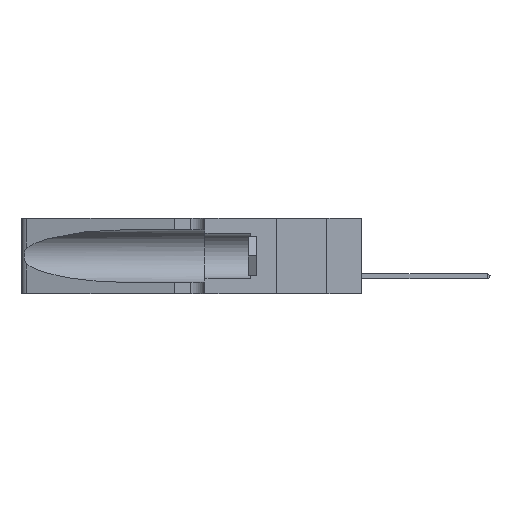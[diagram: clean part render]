
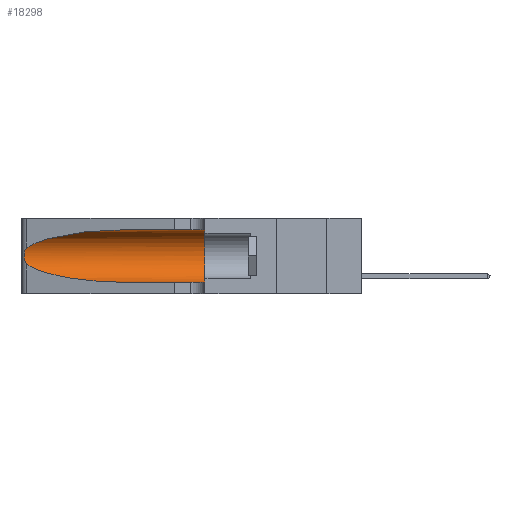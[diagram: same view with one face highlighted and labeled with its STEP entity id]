
A CAD part, left-side view. The second image highlights one B-rep face of the part: STEP entity #18298.
In plain terms, the highlighted cylindrical face has radius 3.308 mm (diameter 6.617 mm), a partial arc.
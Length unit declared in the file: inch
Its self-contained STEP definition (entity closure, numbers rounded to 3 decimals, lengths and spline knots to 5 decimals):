
#325 = DIRECTION ( 'NONE',  ( 0., -1., 0. ) ) ;
#591 = DIRECTION ( 'NONE',  ( 0., 1., 0. ) ) ;
#766 = ORIENTED_EDGE ( 'NONE', *, *, #35172, .T. ) ;
#852 = CARTESIAN_POINT ( 'NONE',  ( 0.25787, 1.23484, 0.2124 ) ) ;
#1067 = CARTESIAN_POINT ( 'NONE',  ( 0.1305, 1.61858, 0.05475 ) ) ;
#1559 = DIRECTION ( 'NONE',  ( 0., -1., 0. ) ) ;
#2289 = VERTEX_POINT ( 'NONE', #9120 ) ;
#2767 = CARTESIAN_POINT ( 'NONE',  ( 0.1305, 1.61858, 0.185 ) ) ;
#3626 = CARTESIAN_POINT ( 'NONE',  ( 0.25856, 1.23593, 0.16098 ) ) ;
#3762 = CARTESIAN_POINT ( 'NONE',  ( 0.25555, 1.22993, 0.14849 ) ) ;
#3997 = CARTESIAN_POINT ( 'NONE',  ( 0.25487, 1.22718, 0.14631 ) ) ;
#4197 = CARTESIAN_POINT ( 'NONE',  ( 0.25487, 1.22718, 0.22369 ) ) ;
#5621 = B_SPLINE_CURVE_WITH_KNOTS ( 'NONE', 3,
 ( #35063, #23959, #24080, #852, #24212, #26990, #6824, #27115, #29912, #3626, #15355, #6574, #3762, #3997 ),
 .UNSPECIFIED., .F., .F.,
 ( 4, 2, 2, 2, 2, 2, 4 ),
 ( 0., 0.00027, 0.00053, 0.00107, 0.0016, 0.00187, 0.00214 ),
 .UNSPECIFIED. ) ;
#6574 = CARTESIAN_POINT ( 'NONE',  ( 0.25639, 1.23186, 0.15144 ) ) ;
#6824 = CARTESIAN_POINT ( 'NONE',  ( 0.26075, 1.23896, 0.19203 ) ) ;
#7132 = CARTESIAN_POINT ( 'NONE',  ( 0.18966, 0.96281, 0.31525 ) ) ;
#7802 = ORIENTED_EDGE ( 'NONE', *, *, #27422, .F. ) ;
#8038 = CARTESIAN_POINT ( 'NONE',  ( 0.25487, 1.22718, 0.14631 ) ) ;
#8056 = LINE ( 'NONE', #1067, #30304 ) ;
#8158 = CARTESIAN_POINT ( 'NONE',  ( 0.1305, 0.72297, 0.05475 ) ) ;
#9120 = CARTESIAN_POINT ( 'NONE',  ( 0.1305, 0.72297, 0.05475 ) ) ;
#9625 = AXIS2_PLACEMENT_3D ( 'NONE', #2767, #325, #32314 ) ;
#10838 = CARTESIAN_POINT ( 'NONE',  ( 0.18966, 0.96281, 0.05475 ) ) ;
#10962 = CARTESIAN_POINT ( 'NONE',  ( 0.2373, 1.15595, 0.08982 ) ) ;
#11157 = EDGE_CURVE ( 'NONE', #15768, #31867, #32030, .T. ) ;
#11395 = VERTEX_POINT ( 'NONE', #28907 ) ;
#12294 = DIRECTION ( 'NONE',  ( 0., 0., 1. ) ) ;
#14663 = EDGE_CURVE ( 'NONE', #11395, #24641, #5621, .T. ) ;
#14729 = EDGE_LOOP ( 'NONE', ( #766, #20952, #30066, #19445, #36388, #7802 ) ) ;
#15355 = CARTESIAN_POINT ( 'NONE',  ( 0.25789, 1.23486, 0.15765 ) ) ;
#15637 = CARTESIAN_POINT ( 'NONE',  ( 0.1305, 0.35, 0.185 ) ) ;
#15768 = VERTEX_POINT ( 'NONE', #24350 ) ;
#17524 = EDGE_CURVE ( 'NONE', #2289, #31867, #8056, .T. ) ;
#18298 = ADVANCED_FACE ( 'NONE', ( #36578 ), #22974, .F. ) ;
#19445 = ORIENTED_EDGE ( 'NONE', *, *, #17524, .T. ) ;
#19544 = CARTESIAN_POINT ( 'NONE',  ( 0.1305, 0.72297, 0.31525 ) ) ;
#20952 = ORIENTED_EDGE ( 'NONE', *, *, #14663, .T. ) ;
#21507 = CARTESIAN_POINT ( 'NONE',  ( 0.1305, 1.61858, 0.31525 ) ) ;
#22389 = CARTESIAN_POINT ( 'NONE',  ( 0.1305, 0.35, 0.05475 ) ) ;
#22974 = CYLINDRICAL_SURFACE ( 'NONE', #9625, 0.13025 ) ;
#23550 =( BOUNDED_CURVE ( )  B_SPLINE_CURVE ( 3, ( #33258, #7132, #36565, #4197 ),
 .UNSPECIFIED., .F., .F. ) 
 B_SPLINE_CURVE_WITH_KNOTS ( ( 4, 4 ),
 ( 1.5708, 2.84003 ),
 .UNSPECIFIED. ) 
 CURVE ( )  GEOMETRIC_REPRESENTATION_ITEM ( )  RATIONAL_B_SPLINE_CURVE ( ( 1., 0.87, 0.87, 1. ) ) 
 REPRESENTATION_ITEM ( '' )  );
#23959 = CARTESIAN_POINT ( 'NONE',  ( 0.25555, 1.22994, 0.2215 ) ) ;
#24080 = CARTESIAN_POINT ( 'NONE',  ( 0.25639, 1.23184, 0.21858 ) ) ;
#24212 = CARTESIAN_POINT ( 'NONE',  ( 0.25854, 1.2359, 0.20912 ) ) ;
#24350 = CARTESIAN_POINT ( 'NONE',  ( 0.1305, 0.35, 0.31525 ) ) ;
#24641 = VERTEX_POINT ( 'NONE', #8038 ) ;
#25293 = CARTESIAN_POINT ( 'NONE',  ( 0.25487, 1.22718, 0.14631 ) ) ;
#25836 = AXIS2_PLACEMENT_3D ( 'NONE', #15637, #591, #12294 ) ;
#26990 = CARTESIAN_POINT ( 'NONE',  ( 0.26018, 1.23835, 0.19895 ) ) ;
#27115 = CARTESIAN_POINT ( 'NONE',  ( 0.26075, 1.23896, 0.178 ) ) ;
#27422 = EDGE_CURVE ( 'NONE', #27460, #15768, #36400, .T. ) ;
#27460 = VERTEX_POINT ( 'NONE', #19544 ) ;
#28907 = CARTESIAN_POINT ( 'NONE',  ( 0.25487, 1.22718, 0.22369 ) ) ;
#29912 = CARTESIAN_POINT ( 'NONE',  ( 0.26017, 1.23833, 0.17102 ) ) ;
#30066 = ORIENTED_EDGE ( 'NONE', *, *, #32873, .T. ) ;
#30300 =( BOUNDED_CURVE ( )  B_SPLINE_CURVE ( 3, ( #25293, #10962, #10838, #8158 ),
 .UNSPECIFIED., .F., .F. ) 
 B_SPLINE_CURVE_WITH_KNOTS ( ( 4, 4 ),
 ( 3.44316, 4.71239 ),
 .UNSPECIFIED. ) 
 CURVE ( )  GEOMETRIC_REPRESENTATION_ITEM ( )  RATIONAL_B_SPLINE_CURVE ( ( 1., 0.87, 0.87, 1. ) ) 
 REPRESENTATION_ITEM ( '' )  );
#30304 = VECTOR ( 'NONE', #1559, 39.37008 ) ;
#30375 = DIRECTION ( 'NONE',  ( 0., -1., 0. ) ) ;
#31867 = VERTEX_POINT ( 'NONE', #22389 ) ;
#32030 = CIRCLE ( 'NONE', #25836, 0.13025 ) ;
#32314 = DIRECTION ( 'NONE',  ( 0., 0., -1. ) ) ;
#32873 = EDGE_CURVE ( 'NONE', #24641, #2289, #30300, .T. ) ;
#33258 = CARTESIAN_POINT ( 'NONE',  ( 0.1305, 0.72297, 0.31525 ) ) ;
#35063 = CARTESIAN_POINT ( 'NONE',  ( 0.25487, 1.22718, 0.22369 ) ) ;
#35172 = EDGE_CURVE ( 'NONE', #27460, #11395, #23550, .T. ) ;
#36388 = ORIENTED_EDGE ( 'NONE', *, *, #11157, .F. ) ;
#36400 = LINE ( 'NONE', #21507, #37264 ) ;
#36565 = CARTESIAN_POINT ( 'NONE',  ( 0.2373, 1.15595, 0.28018 ) ) ;
#36578 = FACE_OUTER_BOUND ( 'NONE', #14729, .T. ) ;
#37264 = VECTOR ( 'NONE', #30375, 39.37008 ) ;
